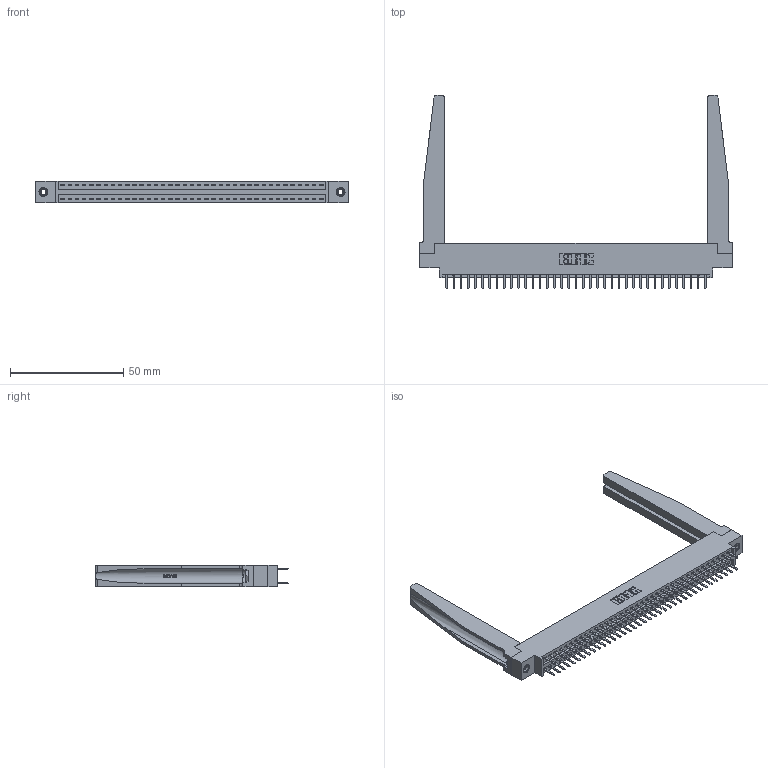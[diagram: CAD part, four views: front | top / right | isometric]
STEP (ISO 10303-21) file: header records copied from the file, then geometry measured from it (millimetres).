
FILE_DESCRIPTION (( 'STEP AP203' ), '1' );
FILE_NAME ('346-074-520-878.STEP', '2022-05-25T01:47:39', ( '' ), ( '' ), 'SwSTEP 2.0', 'SolidWorks 2020', '' );
FILE_SCHEMA (( 'CONFIG_CONTROL_DESIGN' ));
Length unit declared in the file: inch
Products named in the file (5): 345-250-001_345-250-001-102; 346 Part_0.170 Offset - 0.156 Dia-TH; 345-292-001_345-293-120; 346-220-078_345-220-078; 346-074-520-878
Assembly tree (79 placements, depth 2):
  346-074-520-878
    346 Part_0.170 Offset - 0.156 Dia-TH
    345-292-001_345-293-120  x74
    346-220-078_345-220-078  x2
    345-250-001_345-250-001-102  x2
Bounding box: 138.05 x 85.29 x 9.4 mm (x, y, z)
Volume: 20126.3 mm3; surface area: 24765.1 mm2
Topology: 79 solids, 79 shells, 4518 faces, 13047 edges, 8490 vertices
Faces by surface type: plane 2974, cylinder 1492, bspline 36, cone 12, torus 4
Entity records: 30230 total; most frequent: CARTESIAN_POINT 5945, ORIENTED_EDGE 4754, DIRECTION 4263, EDGE_CURVE 2377, VECTOR 1999, LINE 1999, VERTEX_POINT 1576, AXIS2_PLACEMENT_3D 1132
